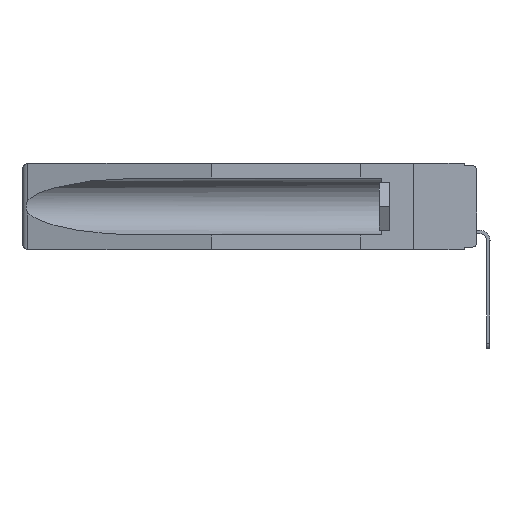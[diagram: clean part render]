
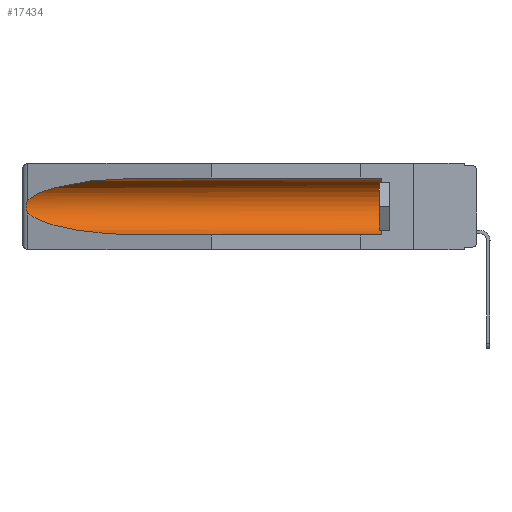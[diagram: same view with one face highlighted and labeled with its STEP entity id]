
A CAD part, left-side view. The second image highlights one B-rep face of the part: STEP entity #17434.
In plain terms, the highlighted cylindrical face has radius 2.857 mm (diameter 5.715 mm), a partial arc.
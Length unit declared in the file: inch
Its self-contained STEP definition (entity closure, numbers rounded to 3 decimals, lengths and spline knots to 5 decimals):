
#682 = CARTESIAN_POINT ( 'NONE',  ( 0.26537, 1.52718, -0.14972 ) ) ;
#1905 = EDGE_CURVE ( 'NONE', #19119, #18373, #21670, .T. ) ;
#2070 = FACE_OUTER_BOUND ( 'NONE', #9003, .T. ) ;
#3034 =( BOUNDED_CURVE ( )  B_SPLINE_CURVE ( 3, ( #21617, #15504, #23106, #6637 ),
 .UNSPECIFIED., .F., .F. ) 
 B_SPLINE_CURVE_WITH_KNOTS ( ( 4, 4 ),
 ( 0.1948, 1.5708 ),
 .UNSPECIFIED. ) 
 CURVE ( )  GEOMETRIC_REPRESENTATION_ITEM ( )  RATIONAL_B_SPLINE_CURVE ( ( 1., 0.848, 0.848, 1. ) ) 
 REPRESENTATION_ITEM ( '' )  );
#3070 = DIRECTION ( 'NONE',  ( 0., 1., 0. ) ) ;
#3097 = EDGE_CURVE ( 'NONE', #15598, #14919, #14410, .T. ) ;
#3390 = ORIENTED_EDGE ( 'NONE', *, *, #18255, .T. ) ;
#4232 = VECTOR ( 'NONE', #3070, 39.37008 ) ;
#4405 = CARTESIAN_POINT ( 'NONE',  ( 0.2675, 1.53308, -0.16763 ) ) ;
#5138 = DIRECTION ( 'NONE',  ( 0., 0., 1. ) ) ;
#5934 = DIRECTION ( 'NONE',  ( 0., 0., 1. ) ) ;
#6384 = VERTEX_POINT ( 'NONE', #17581 ) ;
#6478 = CARTESIAN_POINT ( 'NONE',  ( 0.155, 0.126, -0.059 ) ) ;
#6531 = CARTESIAN_POINT ( 'NONE',  ( 0.26597, 1.52961, -0.15275 ) ) ;
#6621 = CARTESIAN_POINT ( 'NONE',  ( 0.155, 1.07973, -0.059 ) ) ;
#6637 = CARTESIAN_POINT ( 'NONE',  ( 0.155, 1.07973, -0.284 ) ) ;
#7446 = CARTESIAN_POINT ( 'NONE',  ( 0.26537, 1.52718, -0.14972 ) ) ;
#8044 = CARTESIAN_POINT ( 'NONE',  ( 0.26537, 1.52718, -0.19328 ) ) ;
#8415 = CARTESIAN_POINT ( 'NONE',  ( 0.2675, 1.53308, -0.17534 ) ) ;
#8578 = EDGE_CURVE ( 'NONE', #14919, #19119, #14836, .T. ) ;
#9003 = EDGE_LOOP ( 'NONE', ( #10731, #16174, #11071, #10344, #3390, #13777 ) ) ;
#9435 = DIRECTION ( 'NONE',  ( 0., 1., 0. ) ) ;
#10344 = ORIENTED_EDGE ( 'NONE', *, *, #22580, .F. ) ;
#10731 = ORIENTED_EDGE ( 'NONE', *, *, #8578, .T. ) ;
#10950 = LINE ( 'NONE', #24192, #16826 ) ;
#11071 = ORIENTED_EDGE ( 'NONE', *, *, #18153, .T. ) ;
#12013 = CARTESIAN_POINT ( 'NONE',  ( 0.26655, 1.53094, -0.18657 ) ) ;
#12737 = AXIS2_PLACEMENT_3D ( 'NONE', #16130, #14364, #5138 ) ;
#13181 = CARTESIAN_POINT ( 'NONE',  ( 0.155, -0.30754, -0.1715 ) ) ;
#13763 = CARTESIAN_POINT ( 'NONE',  ( 0.2673, 1.5327, -0.16383 ) ) ;
#13777 = ORIENTED_EDGE ( 'NONE', *, *, #3097, .T. ) ;
#13906 = CARTESIAN_POINT ( 'NONE',  ( 0.155, 1.07973, -0.284 ) ) ;
#14364 = DIRECTION ( 'NONE',  ( 0., -1., 0. ) ) ;
#14410 = LINE ( 'NONE', #22134, #4232 ) ;
#14836 =( BOUNDED_CURVE ( )  B_SPLINE_CURVE ( 3, ( #6621, #18459, #16352, #19966 ),
 .UNSPECIFIED., .F., .F. ) 
 B_SPLINE_CURVE_WITH_KNOTS ( ( 4, 4 ),
 ( 4.71239, 6.08839 ),
 .UNSPECIFIED. ) 
 CURVE ( )  GEOMETRIC_REPRESENTATION_ITEM ( )  RATIONAL_B_SPLINE_CURVE ( ( 1., 0.848, 0.848, 1. ) ) 
 REPRESENTATION_ITEM ( '' )  );
#14919 = VERTEX_POINT ( 'NONE', #20854 ) ;
#15504 = CARTESIAN_POINT ( 'NONE',  ( 0.25451, 1.48313, -0.24835 ) ) ;
#15598 = VERTEX_POINT ( 'NONE', #6478 ) ;
#16130 = CARTESIAN_POINT ( 'NONE',  ( 0.155, 0.126, -0.1715 ) ) ;
#16140 = CARTESIAN_POINT ( 'NONE',  ( 0.26597, 1.5296, -0.19026 ) ) ;
#16174 = ORIENTED_EDGE ( 'NONE', *, *, #1905, .T. ) ;
#16352 = CARTESIAN_POINT ( 'NONE',  ( 0.25451, 1.48313, -0.09465 ) ) ;
#16826 = VECTOR ( 'NONE', #18570, 39.37008 ) ;
#17136 = CIRCLE ( 'NONE', #12737, 0.1125 ) ;
#17434 = ADVANCED_FACE ( 'NONE', ( #2070 ), #24531, .F. ) ;
#17581 = CARTESIAN_POINT ( 'NONE',  ( 0.155, 0.126, -0.284 ) ) ;
#18153 = EDGE_CURVE ( 'NONE', #18373, #22053, #3034, .T. ) ;
#18255 = EDGE_CURVE ( 'NONE', #6384, #15598, #17136, .T. ) ;
#18373 = VERTEX_POINT ( 'NONE', #18857 ) ;
#18459 = CARTESIAN_POINT ( 'NONE',  ( 0.21114, 1.30732, -0.059 ) ) ;
#18570 = DIRECTION ( 'NONE',  ( 0., 1., 0. ) ) ;
#18857 = CARTESIAN_POINT ( 'NONE',  ( 0.26537, 1.52718, -0.19328 ) ) ;
#19119 = VERTEX_POINT ( 'NONE', #7446 ) ;
#19754 = CARTESIAN_POINT ( 'NONE',  ( 0.26654, 1.53092, -0.15636 ) ) ;
#19966 = CARTESIAN_POINT ( 'NONE',  ( 0.26537, 1.52718, -0.14972 ) ) ;
#20854 = CARTESIAN_POINT ( 'NONE',  ( 0.155, 1.07973, -0.059 ) ) ;
#21617 = CARTESIAN_POINT ( 'NONE',  ( 0.26537, 1.52718, -0.19328 ) ) ;
#21670 = B_SPLINE_CURVE_WITH_KNOTS ( 'NONE', 3,
 ( #682, #6531, #19754, #13763, #4405, #8415, #21756, #12013, #16140, #8044 ),
 .UNSPECIFIED., .F., .F.,
 ( 4, 2, 2, 2, 4 ),
 ( 0., 0.00029, 0.00058, 0.00087, 0.00117 ),
 .UNSPECIFIED. ) ;
#21756 = CARTESIAN_POINT ( 'NONE',  ( 0.2673, 1.53269, -0.17917 ) ) ;
#22053 = VERTEX_POINT ( 'NONE', #13906 ) ;
#22134 = CARTESIAN_POINT ( 'NONE',  ( 0.155, -0.30754, -0.059 ) ) ;
#22580 = EDGE_CURVE ( 'NONE', #6384, #22053, #10950, .T. ) ;
#22656 = AXIS2_PLACEMENT_3D ( 'NONE', #13181, #9435, #5934 ) ;
#23106 = CARTESIAN_POINT ( 'NONE',  ( 0.21114, 1.30732, -0.284 ) ) ;
#24192 = CARTESIAN_POINT ( 'NONE',  ( 0.155, -0.30754, -0.284 ) ) ;
#24531 = CYLINDRICAL_SURFACE ( 'NONE', #22656, 0.1125 ) ;
